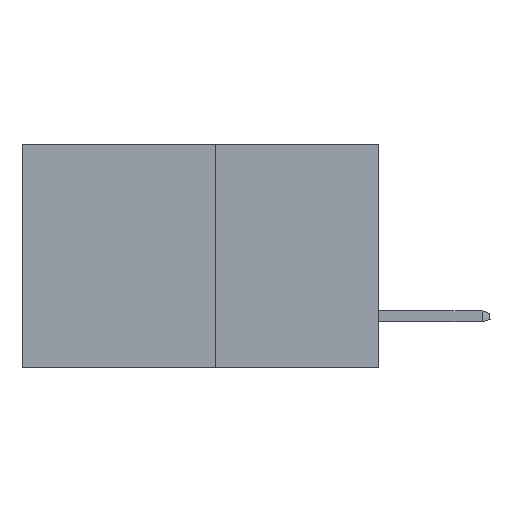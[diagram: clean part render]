
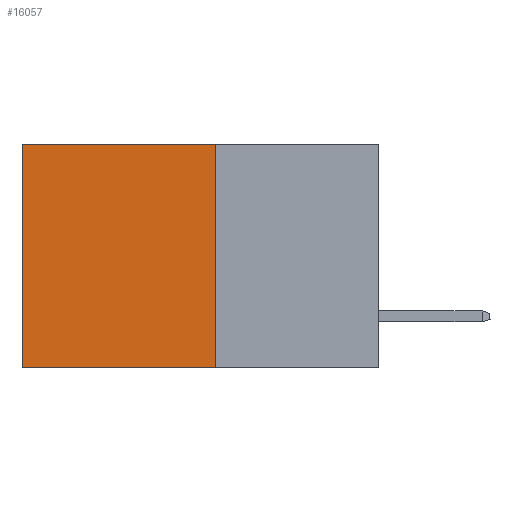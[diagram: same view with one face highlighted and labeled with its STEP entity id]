
A CAD part, left-side view. The second image highlights one B-rep face of the part: STEP entity #16057.
In plain terms, the highlighted planar face has unit normal (-1, 0, 0).
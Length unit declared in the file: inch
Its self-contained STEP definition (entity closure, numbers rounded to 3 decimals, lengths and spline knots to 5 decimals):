
#3 = VECTOR ( 'NONE', #1694, 39.37008 ) ;
#738 = DIRECTION ( 'NONE',  ( 1., 0., 0. ) ) ;
#789 = ORIENTED_EDGE ( 'NONE', *, *, #2479, .T. ) ;
#1530 = VERTEX_POINT ( 'NONE', #14121 ) ;
#1694 = DIRECTION ( 'NONE',  ( 0., 1., 0. ) ) ;
#1698 = VECTOR ( 'NONE', #14716, 39.37008 ) ;
#2214 = VERTEX_POINT ( 'NONE', #2795 ) ;
#2479 = EDGE_CURVE ( 'NONE', #21464, #2214, #11067, .T. ) ;
#2795 = CARTESIAN_POINT ( 'NONE',  ( 0.277, 0.59, -0.37 ) ) ;
#3444 = CARTESIAN_POINT ( 'NONE',  ( 0.277, 0.59, 0. ) ) ;
#3907 = LINE ( 'NONE', #20704, #7946 ) ;
#4559 = CARTESIAN_POINT ( 'NONE',  ( 0.277, 0.27, 0. ) ) ;
#5196 = ORIENTED_EDGE ( 'NONE', *, *, #18809, .F. ) ;
#6074 = CARTESIAN_POINT ( 'NONE',  ( 0.277, 0.27, 0. ) ) ;
#6579 = EDGE_CURVE ( 'NONE', #11513, #1530, #3907, .T. ) ;
#7946 = VECTOR ( 'NONE', #20640, 39.37008 ) ;
#8172 = EDGE_CURVE ( 'NONE', #11513, #21464, #19805, .T. ) ;
#9189 = LINE ( 'NONE', #18208, #3 ) ;
#9935 = ORIENTED_EDGE ( 'NONE', *, *, #6579, .F. ) ;
#10877 = DIRECTION ( 'NONE',  ( 0., 0., -1. ) ) ;
#10972 = AXIS2_PLACEMENT_3D ( 'NONE', #21096, #738, #12764 ) ;
#11055 = PLANE ( 'NONE',  #10972 ) ;
#11067 = LINE ( 'NONE', #11157, #15560 ) ;
#11157 = CARTESIAN_POINT ( 'NONE',  ( 0.277, 0.59, -0.37 ) ) ;
#11513 = VERTEX_POINT ( 'NONE', #4559 ) ;
#12587 = EDGE_LOOP ( 'NONE', ( #789, #5196, #9935, #13208 ) ) ;
#12764 = DIRECTION ( 'NONE',  ( 0., 0., -1. ) ) ;
#13208 = ORIENTED_EDGE ( 'NONE', *, *, #8172, .T. ) ;
#13367 = FACE_OUTER_BOUND ( 'NONE', #12587, .T. ) ;
#14121 = CARTESIAN_POINT ( 'NONE',  ( 0.277, 0.27, -0.37 ) ) ;
#14716 = DIRECTION ( 'NONE',  ( 0., 1., 0. ) ) ;
#15560 = VECTOR ( 'NONE', #10877, 39.37008 ) ;
#16057 = ADVANCED_FACE ( 'NONE', ( #13367 ), #11055, .F. ) ;
#18208 = CARTESIAN_POINT ( 'NONE',  ( 0.277, 0.27, -0.37 ) ) ;
#18809 = EDGE_CURVE ( 'NONE', #1530, #2214, #9189, .T. ) ;
#19805 = LINE ( 'NONE', #6074, #1698 ) ;
#20640 = DIRECTION ( 'NONE',  ( 0., 0., -1. ) ) ;
#20704 = CARTESIAN_POINT ( 'NONE',  ( 0.277, 0.27, -0.37 ) ) ;
#21096 = CARTESIAN_POINT ( 'NONE',  ( 0.277, 0.27, -0.37 ) ) ;
#21464 = VERTEX_POINT ( 'NONE', #3444 ) ;
